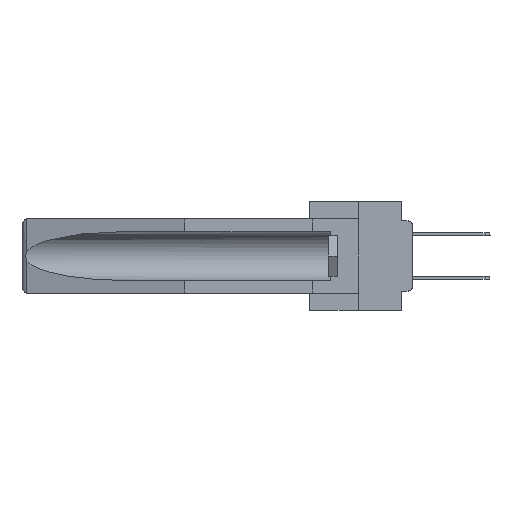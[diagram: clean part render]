
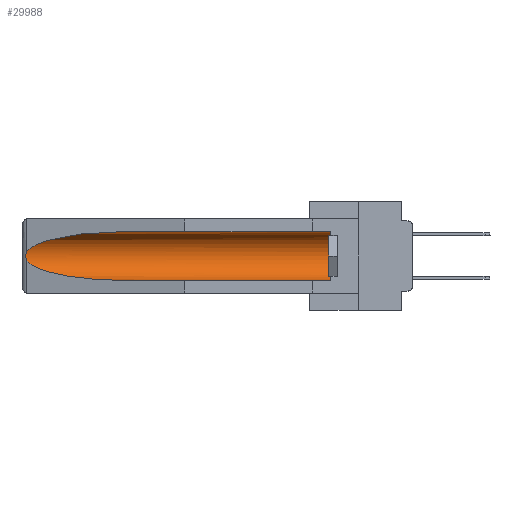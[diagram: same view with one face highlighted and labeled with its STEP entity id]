
A CAD part, left-side view. The second image highlights one B-rep face of the part: STEP entity #29988.
In plain terms, the highlighted cylindrical face has radius 2.857 mm (diameter 5.715 mm), a partial arc.
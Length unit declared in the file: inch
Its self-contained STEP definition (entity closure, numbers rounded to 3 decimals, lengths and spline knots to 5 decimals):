
#686 = CARTESIAN_POINT ( 'NONE',  ( 0.26537, 1.52718, -0.19328 ) ) ;
#1069 = CARTESIAN_POINT ( 'NONE',  ( 0.155, -0.30754, -0.284 ) ) ;
#1483 = LINE ( 'NONE', #18394, #7770 ) ;
#2029 = CARTESIAN_POINT ( 'NONE',  ( 0.21114, 1.30732, -0.284 ) ) ;
#2136 = CARTESIAN_POINT ( 'NONE',  ( 0.25451, 1.48313, -0.24835 ) ) ;
#3690 = CYLINDRICAL_SURFACE ( 'NONE', #11515, 0.1125 ) ;
#3977 =( BOUNDED_CURVE ( )  B_SPLINE_CURVE ( 3, ( #27672, #30043, #15938, #27766 ),
 .UNSPECIFIED., .F., .F. ) 
 B_SPLINE_CURVE_WITH_KNOTS ( ( 4, 4 ),
 ( 4.71239, 6.08839 ),
 .UNSPECIFIED. ) 
 CURVE ( )  GEOMETRIC_REPRESENTATION_ITEM ( )  RATIONAL_B_SPLINE_CURVE ( ( 1., 0.848, 0.848, 1. ) ) 
 REPRESENTATION_ITEM ( '' )  );
#4819 = CARTESIAN_POINT ( 'NONE',  ( 0.26537, 1.52718, -0.14972 ) ) ;
#4974 = ORIENTED_EDGE ( 'NONE', *, *, #12731, .F. ) ;
#5604 = DIRECTION ( 'NONE',  ( 0., 1., 0. ) ) ;
#5828 = VERTEX_POINT ( 'NONE', #686 ) ;
#6008 = CARTESIAN_POINT ( 'NONE',  ( 0.155, 0.126, -0.059 ) ) ;
#6421 = VERTEX_POINT ( 'NONE', #7343 ) ;
#7063 = CARTESIAN_POINT ( 'NONE',  ( 0.2675, 1.53308, -0.17534 ) ) ;
#7146 = LINE ( 'NONE', #1069, #21597 ) ;
#7262 = CARTESIAN_POINT ( 'NONE',  ( 0.26537, 1.52718, -0.19328 ) ) ;
#7343 = CARTESIAN_POINT ( 'NONE',  ( 0.26537, 1.52718, -0.14972 ) ) ;
#7530 =( BOUNDED_CURVE ( )  B_SPLINE_CURVE ( 3, ( #16242, #2136, #2029, #30539 ),
 .UNSPECIFIED., .F., .F. ) 
 B_SPLINE_CURVE_WITH_KNOTS ( ( 4, 4 ),
 ( 0.1948, 1.5708 ),
 .UNSPECIFIED. ) 
 CURVE ( )  GEOMETRIC_REPRESENTATION_ITEM ( )  RATIONAL_B_SPLINE_CURVE ( ( 1., 0.848, 0.848, 1. ) ) 
 REPRESENTATION_ITEM ( '' )  );
#7620 = DIRECTION ( 'NONE',  ( 0., -1., 0. ) ) ;
#7722 = VERTEX_POINT ( 'NONE', #6008 ) ;
#7770 = VECTOR ( 'NONE', #13583, 39.37008 ) ;
#8079 = EDGE_CURVE ( 'NONE', #5828, #8819, #7530, .T. ) ;
#8819 = VERTEX_POINT ( 'NONE', #23928 ) ;
#10386 = EDGE_CURVE ( 'NONE', #7722, #20073, #1483, .T. ) ;
#11244 = DIRECTION ( 'NONE',  ( 0., 1., 0. ) ) ;
#11515 = AXIS2_PLACEMENT_3D ( 'NONE', #13630, #11244, #27775 ) ;
#11530 = EDGE_CURVE ( 'NONE', #20030, #7722, #28314, .T. ) ;
#12731 = EDGE_CURVE ( 'NONE', #20030, #8819, #7146, .T. ) ;
#12827 = AXIS2_PLACEMENT_3D ( 'NONE', #24500, #7620, #24294 ) ;
#13583 = DIRECTION ( 'NONE',  ( 0., 1., 0. ) ) ;
#13630 = CARTESIAN_POINT ( 'NONE',  ( 0.155, -0.30754, -0.1715 ) ) ;
#13757 = FACE_OUTER_BOUND ( 'NONE', #20242, .T. ) ;
#14004 = CARTESIAN_POINT ( 'NONE',  ( 0.26597, 1.52961, -0.15275 ) ) ;
#14696 = ORIENTED_EDGE ( 'NONE', *, *, #8079, .T. ) ;
#14716 = CARTESIAN_POINT ( 'NONE',  ( 0.155, 0.126, -0.284 ) ) ;
#15938 = CARTESIAN_POINT ( 'NONE',  ( 0.25451, 1.48313, -0.09465 ) ) ;
#16242 = CARTESIAN_POINT ( 'NONE',  ( 0.26537, 1.52718, -0.19328 ) ) ;
#16312 = B_SPLINE_CURVE_WITH_KNOTS ( 'NONE', 3,
 ( #4819, #14004, #25905, #21264, #26211, #7063, #30428, #21368, #28546, #7262 ),
 .UNSPECIFIED., .F., .F.,
 ( 4, 2, 2, 2, 4 ),
 ( 0., 0.00029, 0.00058, 0.00087, 0.00117 ),
 .UNSPECIFIED. ) ;
#16470 = CARTESIAN_POINT ( 'NONE',  ( 0.155, 1.07973, -0.059 ) ) ;
#16909 = EDGE_CURVE ( 'NONE', #20073, #6421, #3977, .T. ) ;
#17372 = ORIENTED_EDGE ( 'NONE', *, *, #16909, .T. ) ;
#18394 = CARTESIAN_POINT ( 'NONE',  ( 0.155, -0.30754, -0.059 ) ) ;
#20030 = VERTEX_POINT ( 'NONE', #14716 ) ;
#20073 = VERTEX_POINT ( 'NONE', #16470 ) ;
#20242 = EDGE_LOOP ( 'NONE', ( #17372, #26876, #14696, #4974, #23539, #23272 ) ) ;
#21264 = CARTESIAN_POINT ( 'NONE',  ( 0.2673, 1.5327, -0.16383 ) ) ;
#21368 = CARTESIAN_POINT ( 'NONE',  ( 0.26655, 1.53094, -0.18657 ) ) ;
#21597 = VECTOR ( 'NONE', #5604, 39.37008 ) ;
#23272 = ORIENTED_EDGE ( 'NONE', *, *, #10386, .T. ) ;
#23539 = ORIENTED_EDGE ( 'NONE', *, *, #11530, .T. ) ;
#23928 = CARTESIAN_POINT ( 'NONE',  ( 0.155, 1.07973, -0.284 ) ) ;
#24294 = DIRECTION ( 'NONE',  ( 0., 0., 1. ) ) ;
#24455 = EDGE_CURVE ( 'NONE', #6421, #5828, #16312, .T. ) ;
#24500 = CARTESIAN_POINT ( 'NONE',  ( 0.155, 0.126, -0.1715 ) ) ;
#25905 = CARTESIAN_POINT ( 'NONE',  ( 0.26654, 1.53092, -0.15636 ) ) ;
#26211 = CARTESIAN_POINT ( 'NONE',  ( 0.2675, 1.53308, -0.16763 ) ) ;
#26876 = ORIENTED_EDGE ( 'NONE', *, *, #24455, .T. ) ;
#27672 = CARTESIAN_POINT ( 'NONE',  ( 0.155, 1.07973, -0.059 ) ) ;
#27766 = CARTESIAN_POINT ( 'NONE',  ( 0.26537, 1.52718, -0.14972 ) ) ;
#27775 = DIRECTION ( 'NONE',  ( 0., 0., 1. ) ) ;
#28314 = CIRCLE ( 'NONE', #12827, 0.1125 ) ;
#28546 = CARTESIAN_POINT ( 'NONE',  ( 0.26597, 1.5296, -0.19026 ) ) ;
#29988 = ADVANCED_FACE ( 'NONE', ( #13757 ), #3690, .F. ) ;
#30043 = CARTESIAN_POINT ( 'NONE',  ( 0.21114, 1.30732, -0.059 ) ) ;
#30428 = CARTESIAN_POINT ( 'NONE',  ( 0.2673, 1.53269, -0.17917 ) ) ;
#30539 = CARTESIAN_POINT ( 'NONE',  ( 0.155, 1.07973, -0.284 ) ) ;
